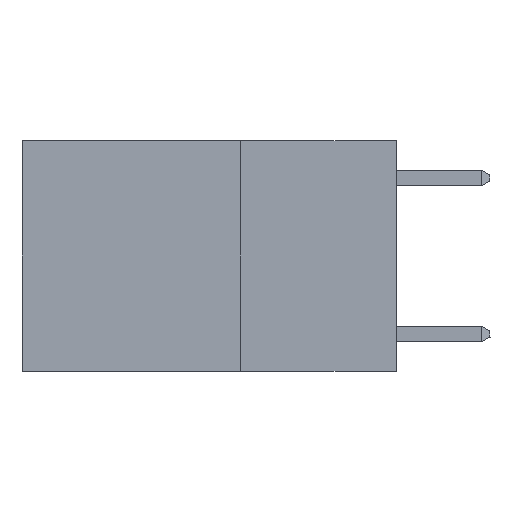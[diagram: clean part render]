
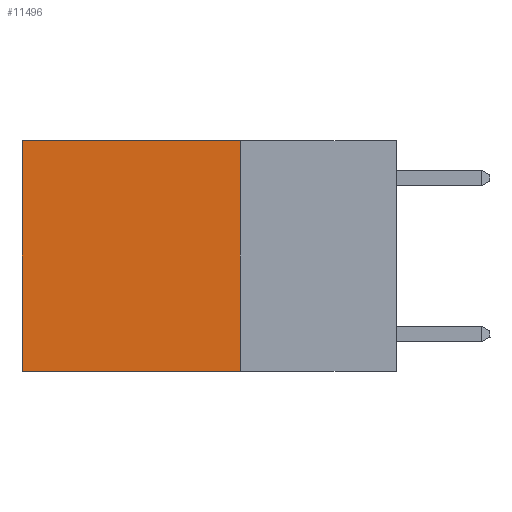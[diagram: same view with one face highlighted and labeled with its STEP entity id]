
A CAD part, left-side view. The second image highlights one B-rep face of the part: STEP entity #11496.
In plain terms, the highlighted planar face has unit normal (-1, 0, 0).
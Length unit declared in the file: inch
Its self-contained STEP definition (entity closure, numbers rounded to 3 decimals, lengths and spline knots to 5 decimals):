
#536 = CARTESIAN_POINT ( 'NONE',  ( 0.2625, 0.25, 0. ) ) ;
#581 = ORIENTED_EDGE ( 'NONE', *, *, #10725, .F. ) ;
#730 = CARTESIAN_POINT ( 'NONE',  ( 0.2625, 0.6, 0. ) ) ;
#779 = VECTOR ( 'NONE', #8104, 39.37008 ) ;
#1758 = ORIENTED_EDGE ( 'NONE', *, *, #5163, .T. ) ;
#2534 = ORIENTED_EDGE ( 'NONE', *, *, #5210, .F. ) ;
#2624 = DIRECTION ( 'NONE',  ( 1., 0., 0. ) ) ;
#2869 = DIRECTION ( 'NONE',  ( 0., 1., 0. ) ) ;
#3053 = EDGE_LOOP ( 'NONE', ( #8792, #2534, #581, #1758 ) ) ;
#3457 = CARTESIAN_POINT ( 'NONE',  ( 0.2625, 0.25, 0. ) ) ;
#3779 = VERTEX_POINT ( 'NONE', #6091 ) ;
#3849 = LINE ( 'NONE', #9898, #779 ) ;
#4158 = LINE ( 'NONE', #9849, #11782 ) ;
#4363 = CARTESIAN_POINT ( 'NONE',  ( 0.2625, 0.25, -0.37 ) ) ;
#4409 = DIRECTION ( 'NONE',  ( 0., 0., -1. ) ) ;
#5163 = EDGE_CURVE ( 'NONE', #3779, #7259, #4158, .T. ) ;
#5210 = EDGE_CURVE ( 'NONE', #7314, #6974, #3849, .T. ) ;
#5387 = VECTOR ( 'NONE', #6737, 39.37008 ) ;
#6069 = AXIS2_PLACEMENT_3D ( 'NONE', #536, #2624, #9623 ) ;
#6091 = CARTESIAN_POINT ( 'NONE',  ( 0.2625, 0.25, 0. ) ) ;
#6593 = PLANE ( 'NONE',  #6069 ) ;
#6737 = DIRECTION ( 'NONE',  ( 0., 0., -1. ) ) ;
#6974 = VERTEX_POINT ( 'NONE', #9852 ) ;
#7259 = VERTEX_POINT ( 'NONE', #8280 ) ;
#7314 = VERTEX_POINT ( 'NONE', #4363 ) ;
#7923 = LINE ( 'NONE', #3457, #10576 ) ;
#8104 = DIRECTION ( 'NONE',  ( 0., 1., 0. ) ) ;
#8280 = CARTESIAN_POINT ( 'NONE',  ( 0.2625, 0.6, 0. ) ) ;
#8347 = LINE ( 'NONE', #730, #5387 ) ;
#8792 = ORIENTED_EDGE ( 'NONE', *, *, #12786, .T. ) ;
#9155 = FACE_OUTER_BOUND ( 'NONE', #3053, .T. ) ;
#9623 = DIRECTION ( 'NONE',  ( 0., 0., -1. ) ) ;
#9849 = CARTESIAN_POINT ( 'NONE',  ( 0.2625, 0.25, 0. ) ) ;
#9852 = CARTESIAN_POINT ( 'NONE',  ( 0.2625, 0.6, -0.37 ) ) ;
#9898 = CARTESIAN_POINT ( 'NONE',  ( 0.2625, 0.25, -0.37 ) ) ;
#10576 = VECTOR ( 'NONE', #4409, 39.37008 ) ;
#10725 = EDGE_CURVE ( 'NONE', #3779, #7314, #7923, .T. ) ;
#11496 = ADVANCED_FACE ( 'NONE', ( #9155 ), #6593, .F. ) ;
#11782 = VECTOR ( 'NONE', #2869, 39.37008 ) ;
#12786 = EDGE_CURVE ( 'NONE', #7259, #6974, #8347, .T. ) ;
